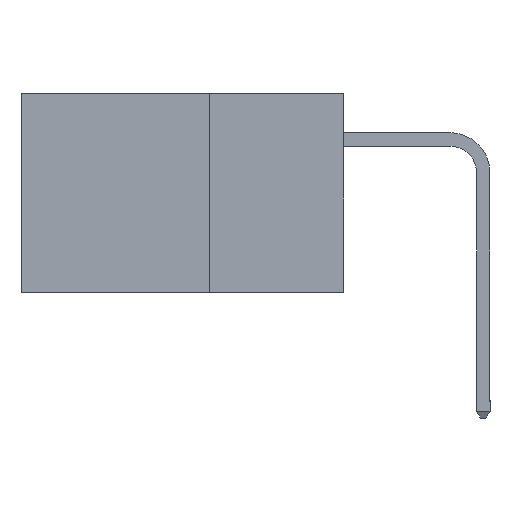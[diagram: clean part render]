
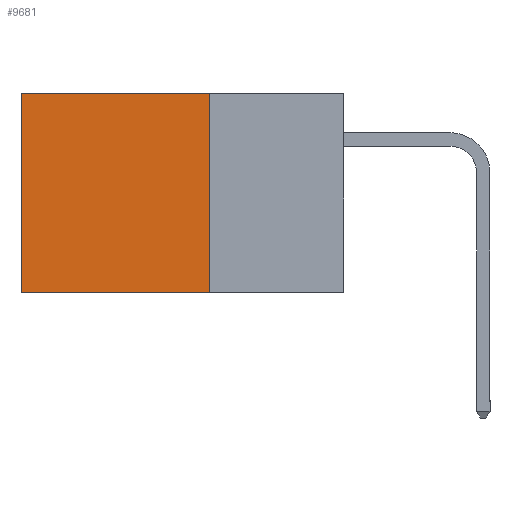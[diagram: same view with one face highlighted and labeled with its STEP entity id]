
A CAD part, left-side view. The second image highlights one B-rep face of the part: STEP entity #9681.
In plain terms, the highlighted planar face has unit normal (-1, 0, 0).
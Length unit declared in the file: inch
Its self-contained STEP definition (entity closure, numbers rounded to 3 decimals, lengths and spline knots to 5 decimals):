
#173 = DIRECTION ( 'NONE',  ( 0., 1., 0. ) ) ;
#214 = CARTESIAN_POINT ( 'NONE',  ( 0.2615, 0.25, 0. ) ) ;
#1168 = DIRECTION ( 'NONE',  ( 0., 0., -1. ) ) ;
#1707 = EDGE_LOOP ( 'NONE', ( #5236, #8758, #4387, #2174 ) ) ;
#1868 = VECTOR ( 'NONE', #173, 39.37008 ) ;
#1898 = VERTEX_POINT ( 'NONE', #9061 ) ;
#2174 = ORIENTED_EDGE ( 'NONE', *, *, #10063, .T. ) ;
#2638 = CARTESIAN_POINT ( 'NONE',  ( 0.2615, 0.25, -0.37 ) ) ;
#2732 = CARTESIAN_POINT ( 'NONE',  ( 0.2615, 0.25, -0.37 ) ) ;
#2740 = CARTESIAN_POINT ( 'NONE',  ( 0.2615, 0.25, -0.37 ) ) ;
#4110 = CARTESIAN_POINT ( 'NONE',  ( 0.2615, 0.6, -0.37 ) ) ;
#4387 = ORIENTED_EDGE ( 'NONE', *, *, #6020, .F. ) ;
#4391 = CARTESIAN_POINT ( 'NONE',  ( 0.2615, 0.25, -0.37 ) ) ;
#4506 = VERTEX_POINT ( 'NONE', #2732 ) ;
#4679 = FACE_OUTER_BOUND ( 'NONE', #1707, .T. ) ;
#4843 = DIRECTION ( 'NONE',  ( 0., 0., -1. ) ) ;
#5109 = LINE ( 'NONE', #2740, #7388 ) ;
#5236 = ORIENTED_EDGE ( 'NONE', *, *, #6424, .T. ) ;
#5625 = VERTEX_POINT ( 'NONE', #214 ) ;
#5677 = CARTESIAN_POINT ( 'NONE',  ( 0.2615, 0.25, 0. ) ) ;
#5946 = EDGE_CURVE ( 'NONE', #4506, #7054, #6551, .T. ) ;
#5957 = DIRECTION ( 'NONE',  ( 1., 0., 0. ) ) ;
#6020 = EDGE_CURVE ( 'NONE', #5625, #4506, #5109, .T. ) ;
#6424 = EDGE_CURVE ( 'NONE', #1898, #7054, #9584, .T. ) ;
#6449 = DIRECTION ( 'NONE',  ( 0., 1., 0. ) ) ;
#6551 = LINE ( 'NONE', #2638, #1868 ) ;
#6958 = VECTOR ( 'NONE', #6449, 39.37008 ) ;
#7054 = VERTEX_POINT ( 'NONE', #4110 ) ;
#7246 = AXIS2_PLACEMENT_3D ( 'NONE', #4391, #5957, #1168 ) ;
#7388 = VECTOR ( 'NONE', #8898, 39.37008 ) ;
#8630 = CARTESIAN_POINT ( 'NONE',  ( 0.2615, 0.6, -0.37 ) ) ;
#8758 = ORIENTED_EDGE ( 'NONE', *, *, #5946, .F. ) ;
#8898 = DIRECTION ( 'NONE',  ( 0., 0., -1. ) ) ;
#8948 = PLANE ( 'NONE',  #7246 ) ;
#9061 = CARTESIAN_POINT ( 'NONE',  ( 0.2615, 0.6, 0. ) ) ;
#9174 = LINE ( 'NONE', #5677, #6958 ) ;
#9339 = VECTOR ( 'NONE', #4843, 39.37008 ) ;
#9584 = LINE ( 'NONE', #8630, #9339 ) ;
#9681 = ADVANCED_FACE ( 'NONE', ( #4679 ), #8948, .F. ) ;
#10063 = EDGE_CURVE ( 'NONE', #5625, #1898, #9174, .T. ) ;
